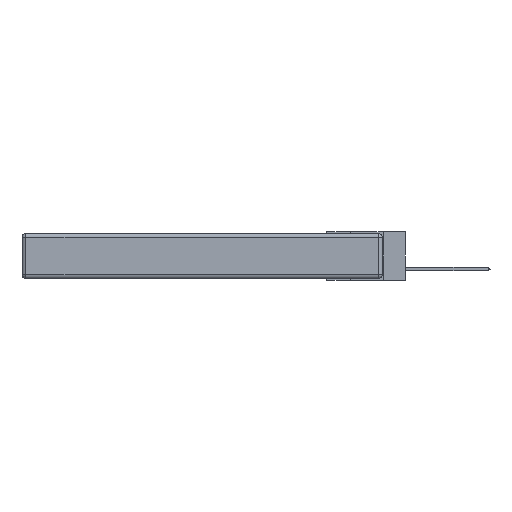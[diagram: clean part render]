
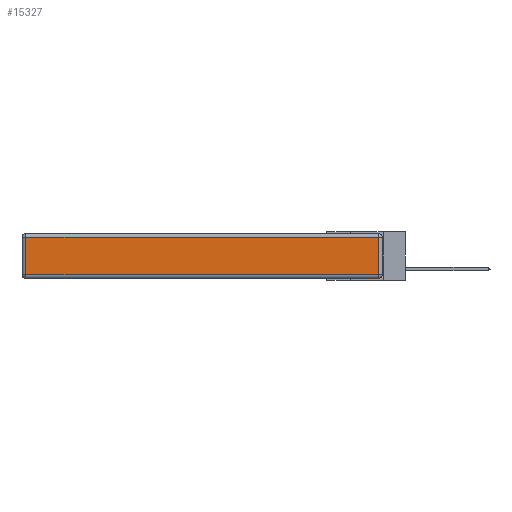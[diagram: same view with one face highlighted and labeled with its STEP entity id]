
A CAD part, left-side view. The second image highlights one B-rep face of the part: STEP entity #15327.
In plain terms, the highlighted planar face has unit normal (-1, 0, 0).
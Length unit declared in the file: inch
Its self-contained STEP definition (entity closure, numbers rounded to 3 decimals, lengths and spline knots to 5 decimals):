
#2061 = CARTESIAN_POINT ( 'NONE',  ( 0., 0., -0.313 ) ) ;
#2230 = DIRECTION ( 'NONE',  ( 0., 0., 1. ) ) ;
#2312 = VERTEX_POINT ( 'NONE', #19357 ) ;
#2396 = AXIS2_PLACEMENT_3D ( 'NONE', #20366, #3459, #20290 ) ;
#2667 = ORIENTED_EDGE ( 'NONE', *, *, #18036, .T. ) ;
#3044 = LINE ( 'NONE', #5269, #16786 ) ;
#3322 = EDGE_CURVE ( 'NONE', #12286, #18552, #20724, .T. ) ;
#3459 = DIRECTION ( 'NONE',  ( -1., 0., 0. ) ) ;
#3777 = DIRECTION ( 'NONE',  ( 0., -1., 0. ) ) ;
#4117 = VECTOR ( 'NONE', #17659, 39.37008 ) ;
#4444 = ORIENTED_EDGE ( 'NONE', *, *, #3322, .T. ) ;
#5269 = CARTESIAN_POINT ( 'NONE',  ( 0., 2.75, -0.03 ) ) ;
#6506 = ORIENTED_EDGE ( 'NONE', *, *, #7569, .T. ) ;
#7248 = FACE_OUTER_BOUND ( 'NONE', #8422, .T. ) ;
#7569 = EDGE_CURVE ( 'NONE', #18552, #10809, #3044, .T. ) ;
#7670 = VECTOR ( 'NONE', #3777, 39.37008 ) ;
#7852 = EDGE_CURVE ( 'NONE', #10809, #2312, #13637, .T. ) ;
#8422 = EDGE_LOOP ( 'NONE', ( #2667, #4444, #6506, #10095 ) ) ;
#10095 = ORIENTED_EDGE ( 'NONE', *, *, #7852, .T. ) ;
#10809 = VERTEX_POINT ( 'NONE', #16879 ) ;
#12070 = CARTESIAN_POINT ( 'NONE',  ( 0., 0.03, -0.343 ) ) ;
#12286 = VERTEX_POINT ( 'NONE', #13388 ) ;
#12813 = VECTOR ( 'NONE', #2230, 39.37008 ) ;
#13388 = CARTESIAN_POINT ( 'NONE',  ( 0., 0.03, -0.313 ) ) ;
#13637 = LINE ( 'NONE', #16070, #4117 ) ;
#13739 = DIRECTION ( 'NONE',  ( 0., 1., 0. ) ) ;
#15327 = ADVANCED_FACE ( 'NONE', ( #7248 ), #16795, .T. ) ;
#16070 = CARTESIAN_POINT ( 'NONE',  ( 0., 2.72, -0.343 ) ) ;
#16786 = VECTOR ( 'NONE', #13739, 39.37008 ) ;
#16795 = PLANE ( 'NONE',  #2396 ) ;
#16879 = CARTESIAN_POINT ( 'NONE',  ( 0., 2.72, -0.03 ) ) ;
#17659 = DIRECTION ( 'NONE',  ( 0., 0., -1. ) ) ;
#18036 = EDGE_CURVE ( 'NONE', #2312, #12286, #19055, .T. ) ;
#18552 = VERTEX_POINT ( 'NONE', #19247 ) ;
#19055 = LINE ( 'NONE', #2061, #7670 ) ;
#19247 = CARTESIAN_POINT ( 'NONE',  ( 0., 0.03, -0.03 ) ) ;
#19357 = CARTESIAN_POINT ( 'NONE',  ( 0., 2.72, -0.313 ) ) ;
#20290 = DIRECTION ( 'NONE',  ( 0., 0., 1. ) ) ;
#20366 = CARTESIAN_POINT ( 'NONE',  ( 0., 0., -0.343 ) ) ;
#20724 = LINE ( 'NONE', #12070, #12813 ) ;
